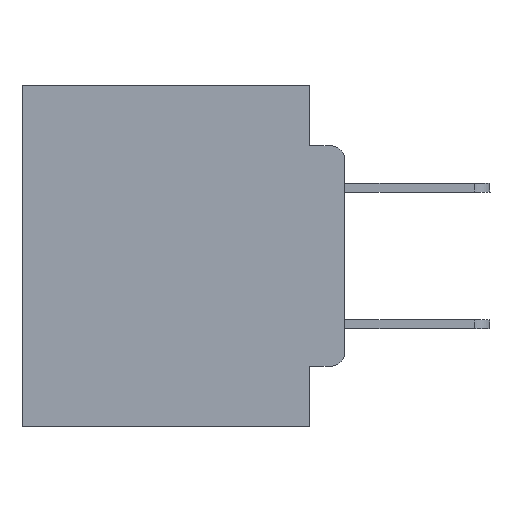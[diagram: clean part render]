
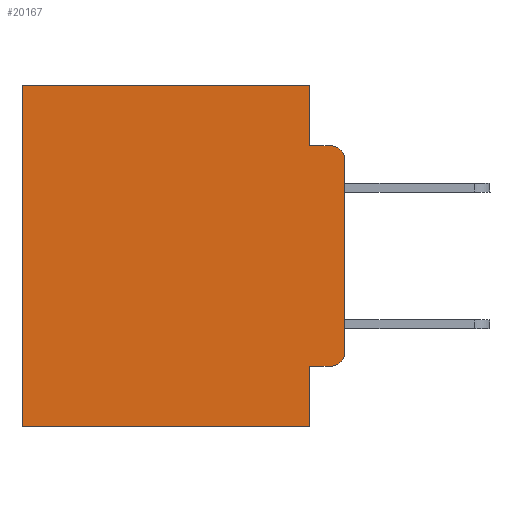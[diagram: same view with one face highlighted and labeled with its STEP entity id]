
A CAD part, left-side view. The second image highlights one B-rep face of the part: STEP entity #20167.
In plain terms, the highlighted planar face has unit normal (-1, 0, 0).
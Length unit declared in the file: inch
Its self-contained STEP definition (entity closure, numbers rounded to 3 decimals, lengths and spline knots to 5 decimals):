
#92 = AXIS2_PLACEMENT_3D ( 'NONE', #20447, #849, #20078 ) ;
#444 = EDGE_CURVE ( 'NONE', #22991, #3275, #6311, .T. ) ;
#849 = DIRECTION ( 'NONE',  ( 1., 0., 0. ) ) ;
#1833 = CARTESIAN_POINT ( 'NONE',  ( 0.298, 0., -0.1085 ) ) ;
#2112 = CARTESIAN_POINT ( 'NONE',  ( 0.298, 0.473, 0. ) ) ;
#2183 = CARTESIAN_POINT ( 'NONE',  ( 0.298, 0.051, 0. ) ) ;
#2539 = CARTESIAN_POINT ( 'NONE',  ( 0.298, 0.02, -0.3915 ) ) ;
#3018 = VERTEX_POINT ( 'NONE', #15464 ) ;
#3156 = DIRECTION ( 'NONE',  ( 0., 0., -1. ) ) ;
#3275 = VERTEX_POINT ( 'NONE', #14560 ) ;
#3631 = CARTESIAN_POINT ( 'NONE',  ( 0.298, 0.051, 0. ) ) ;
#3726 = CIRCLE ( 'NONE', #5373, 0.02 ) ;
#3774 = ORIENTED_EDGE ( 'NONE', *, *, #7577, .T. ) ;
#3968 = DIRECTION ( 'NONE',  ( 0., 0., -1. ) ) ;
#4033 = EDGE_CURVE ( 'NONE', #25374, #3275, #23954, .T. ) ;
#4047 = EDGE_LOOP ( 'NONE', ( #10529, #14745, #23654, #15504, #3774, #13566, #20633, #20426, #27012, #15484 ) ) ;
#4337 = LINE ( 'NONE', #12317, #23844 ) ;
#5333 = LINE ( 'NONE', #14445, #16055 ) ;
#5373 = AXIS2_PLACEMENT_3D ( 'NONE', #22515, #9605, #3156 ) ;
#5384 = EDGE_CURVE ( 'NONE', #3018, #9113, #9063, .T. ) ;
#5498 = VERTEX_POINT ( 'NONE', #2183 ) ;
#5591 = DIRECTION ( 'NONE',  ( 0., 0., -1. ) ) ;
#5692 = VECTOR ( 'NONE', #21368, 39.37008 ) ;
#5846 = EDGE_CURVE ( 'NONE', #5498, #3018, #27623, .T. ) ;
#6098 = CARTESIAN_POINT ( 'NONE',  ( 0.298, 0.051, -0.0885 ) ) ;
#6105 = FACE_OUTER_BOUND ( 'NONE', #4047, .T. ) ;
#6311 = LINE ( 'NONE', #11790, #7310 ) ;
#7310 = VECTOR ( 'NONE', #5591, 39.37008 ) ;
#7554 = CARTESIAN_POINT ( 'NONE',  ( 0.298, 0.02, -0.0885 ) ) ;
#7577 = EDGE_CURVE ( 'NONE', #5498, #13409, #5333, .T. ) ;
#7696 = VERTEX_POINT ( 'NONE', #21008 ) ;
#7965 = DIRECTION ( 'NONE',  ( 0., 1., 0. ) ) ;
#8165 = DIRECTION ( 'NONE',  ( 0., 1., 0. ) ) ;
#8270 = VERTEX_POINT ( 'NONE', #14231 ) ;
#8594 = CARTESIAN_POINT ( 'NONE',  ( 0.298, 0.051, -0.5 ) ) ;
#8779 = DIRECTION ( 'NONE',  ( -1., 0., 0. ) ) ;
#9063 = LINE ( 'NONE', #6098, #19409 ) ;
#9113 = VERTEX_POINT ( 'NONE', #7554 ) ;
#9380 = VECTOR ( 'NONE', #3968, 39.37008 ) ;
#9605 = DIRECTION ( 'NONE',  ( -1., 0., 0. ) ) ;
#10099 = DIRECTION ( 'NONE',  ( 0., 0., -1. ) ) ;
#10529 = ORIENTED_EDGE ( 'NONE', *, *, #444, .F. ) ;
#10673 = DIRECTION ( 'NONE',  ( 0., 0., -1. ) ) ;
#11449 = VECTOR ( 'NONE', #10099, 39.37008 ) ;
#11790 = CARTESIAN_POINT ( 'NONE',  ( 0.298, 0., 0. ) ) ;
#12096 = LINE ( 'NONE', #2112, #9380 ) ;
#12317 = CARTESIAN_POINT ( 'NONE',  ( 0.298, 0., -0.5 ) ) ;
#13036 = LINE ( 'NONE', #24773, #22482 ) ;
#13409 = VERTEX_POINT ( 'NONE', #23388 ) ;
#13566 = ORIENTED_EDGE ( 'NONE', *, *, #21005, .T. ) ;
#14231 = CARTESIAN_POINT ( 'NONE',  ( 0.298, 0.473, -0.5 ) ) ;
#14445 = CARTESIAN_POINT ( 'NONE',  ( 0.298, 0., 0. ) ) ;
#14560 = CARTESIAN_POINT ( 'NONE',  ( 0.298, 0., -0.3915 ) ) ;
#14732 = VERTEX_POINT ( 'NONE', #8594 ) ;
#14745 = ORIENTED_EDGE ( 'NONE', *, *, #25649, .T. ) ;
#15464 = CARTESIAN_POINT ( 'NONE',  ( 0.298, 0.051, -0.0885 ) ) ;
#15484 = ORIENTED_EDGE ( 'NONE', *, *, #4033, .T. ) ;
#15504 = ORIENTED_EDGE ( 'NONE', *, *, #5846, .F. ) ;
#16055 = VECTOR ( 'NONE', #7965, 39.37008 ) ;
#16932 = CARTESIAN_POINT ( 'NONE',  ( 0.298, 0.02, -0.4115 ) ) ;
#19409 = VECTOR ( 'NONE', #21344, 39.37008 ) ;
#20043 = AXIS2_PLACEMENT_3D ( 'NONE', #2539, #8779, #10673 ) ;
#20078 = DIRECTION ( 'NONE',  ( 0., 0., -1. ) ) ;
#20167 = ADVANCED_FACE ( 'NONE', ( #6105 ), #22446, .F. ) ;
#20426 = ORIENTED_EDGE ( 'NONE', *, *, #22877, .F. ) ;
#20447 = CARTESIAN_POINT ( 'NONE',  ( 0.298, 0., 0. ) ) ;
#20633 = ORIENTED_EDGE ( 'NONE', *, *, #23002, .F. ) ;
#20827 = LINE ( 'NONE', #27769, #5692 ) ;
#21005 = EDGE_CURVE ( 'NONE', #13409, #8270, #12096, .T. ) ;
#21008 = CARTESIAN_POINT ( 'NONE',  ( 0.298, 0.051, -0.4115 ) ) ;
#21344 = DIRECTION ( 'NONE',  ( 0., -1., 0. ) ) ;
#21368 = DIRECTION ( 'NONE',  ( 0., -1., 0. ) ) ;
#22446 = PLANE ( 'NONE',  #92 ) ;
#22482 = VECTOR ( 'NONE', #27128, 39.37008 ) ;
#22515 = CARTESIAN_POINT ( 'NONE',  ( 0.298, 0.02, -0.1085 ) ) ;
#22877 = EDGE_CURVE ( 'NONE', #7696, #14732, #13036, .T. ) ;
#22991 = VERTEX_POINT ( 'NONE', #1833 ) ;
#23002 = EDGE_CURVE ( 'NONE', #14732, #8270, #4337, .T. ) ;
#23388 = CARTESIAN_POINT ( 'NONE',  ( 0.298, 0.473, 0. ) ) ;
#23654 = ORIENTED_EDGE ( 'NONE', *, *, #5384, .F. ) ;
#23844 = VECTOR ( 'NONE', #8165, 39.37008 ) ;
#23954 = CIRCLE ( 'NONE', #20043, 0.02 ) ;
#24773 = CARTESIAN_POINT ( 'NONE',  ( 0.298, 0.051, 0. ) ) ;
#25374 = VERTEX_POINT ( 'NONE', #16932 ) ;
#25649 = EDGE_CURVE ( 'NONE', #22991, #9113, #3726, .T. ) ;
#26282 = EDGE_CURVE ( 'NONE', #7696, #25374, #20827, .T. ) ;
#27012 = ORIENTED_EDGE ( 'NONE', *, *, #26282, .T. ) ;
#27128 = DIRECTION ( 'NONE',  ( 0., 0., -1. ) ) ;
#27623 = LINE ( 'NONE', #3631, #11449 ) ;
#27769 = CARTESIAN_POINT ( 'NONE',  ( 0.298, 0.051, -0.4115 ) ) ;
